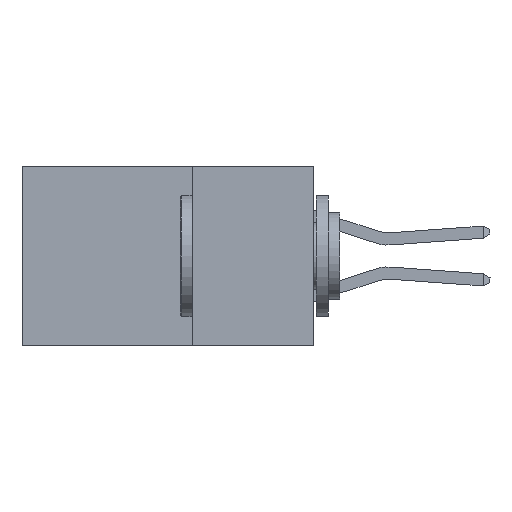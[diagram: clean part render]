
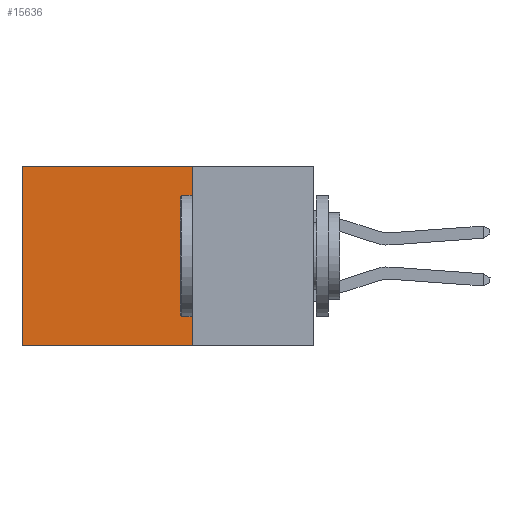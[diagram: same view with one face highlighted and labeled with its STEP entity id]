
A CAD part, left-side view. The second image highlights one B-rep face of the part: STEP entity #15636.
In plain terms, the highlighted planar face has unit normal (-1, 0, 0).
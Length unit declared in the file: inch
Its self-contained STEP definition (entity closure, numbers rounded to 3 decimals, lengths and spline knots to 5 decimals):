
#221 = LINE ( 'NONE', #3701, #13081 ) ;
#1159 = LINE ( 'NONE', #10216, #10324 ) ;
#1638 = EDGE_CURVE ( 'NONE', #11534, #11928, #1159, .T. ) ;
#1771 = DIRECTION ( 'NONE',  ( 0., 0., -1. ) ) ;
#1884 = ORIENTED_EDGE ( 'NONE', *, *, #1638, .T. ) ;
#2621 = AXIS2_PLACEMENT_3D ( 'NONE', #14184, #13975, #11567 ) ;
#2879 = CARTESIAN_POINT ( 'NONE',  ( 0.2875, 0.6, -0.37 ) ) ;
#3299 = FACE_OUTER_BOUND ( 'NONE', #9403, .T. ) ;
#3701 = CARTESIAN_POINT ( 'NONE',  ( 0.2875, 0.25, 0. ) ) ;
#4155 = VERTEX_POINT ( 'NONE', #12236 ) ;
#5351 = ORIENTED_EDGE ( 'NONE', *, *, #9229, .T. ) ;
#6284 = CARTESIAN_POINT ( 'NONE',  ( 0.2875, 0.25, 0. ) ) ;
#6481 = PLANE ( 'NONE',  #2621 ) ;
#7193 = LINE ( 'NONE', #9088, #15004 ) ;
#8181 = VECTOR ( 'NONE', #8632, 39.37008 ) ;
#8368 = LINE ( 'NONE', #9816, #8181 ) ;
#8632 = DIRECTION ( 'NONE',  ( 0., 1., 0. ) ) ;
#9088 = CARTESIAN_POINT ( 'NONE',  ( 0.2875, 0.6, 0. ) ) ;
#9229 = EDGE_CURVE ( 'NONE', #11928, #14448, #7193, .T. ) ;
#9403 = EDGE_LOOP ( 'NONE', ( #5351, #11028, #12996, #1884 ) ) ;
#9816 = CARTESIAN_POINT ( 'NONE',  ( 0.2875, 0.25, -0.37 ) ) ;
#9906 = DIRECTION ( 'NONE',  ( 0., 0., -1. ) ) ;
#10216 = CARTESIAN_POINT ( 'NONE',  ( 0.2875, 0.25, 0. ) ) ;
#10324 = VECTOR ( 'NONE', #10643, 39.37008 ) ;
#10643 = DIRECTION ( 'NONE',  ( 0., 1., 0. ) ) ;
#11028 = ORIENTED_EDGE ( 'NONE', *, *, #15987, .F. ) ;
#11534 = VERTEX_POINT ( 'NONE', #6284 ) ;
#11567 = DIRECTION ( 'NONE',  ( 0., 0., -1. ) ) ;
#11928 = VERTEX_POINT ( 'NONE', #14776 ) ;
#12236 = CARTESIAN_POINT ( 'NONE',  ( 0.2875, 0.25, -0.37 ) ) ;
#12996 = ORIENTED_EDGE ( 'NONE', *, *, #13690, .F. ) ;
#13081 = VECTOR ( 'NONE', #9906, 39.37008 ) ;
#13690 = EDGE_CURVE ( 'NONE', #11534, #4155, #221, .T. ) ;
#13975 = DIRECTION ( 'NONE',  ( 1., 0., 0. ) ) ;
#14184 = CARTESIAN_POINT ( 'NONE',  ( 0.2875, 0.25, 0. ) ) ;
#14448 = VERTEX_POINT ( 'NONE', #2879 ) ;
#14776 = CARTESIAN_POINT ( 'NONE',  ( 0.2875, 0.6, 0. ) ) ;
#15004 = VECTOR ( 'NONE', #1771, 39.37008 ) ;
#15636 = ADVANCED_FACE ( 'NONE', ( #3299 ), #6481, .F. ) ;
#15987 = EDGE_CURVE ( 'NONE', #4155, #14448, #8368, .T. ) ;
